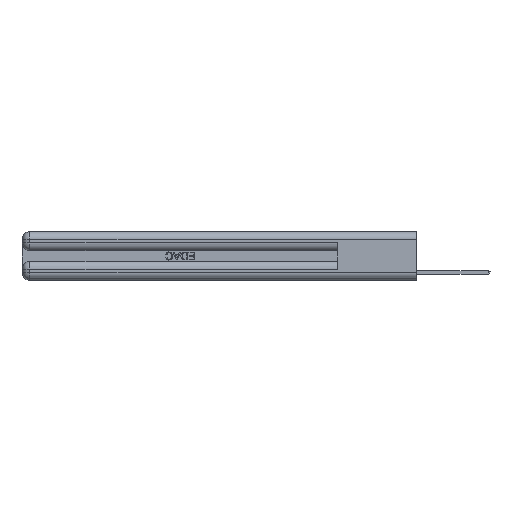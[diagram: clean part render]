
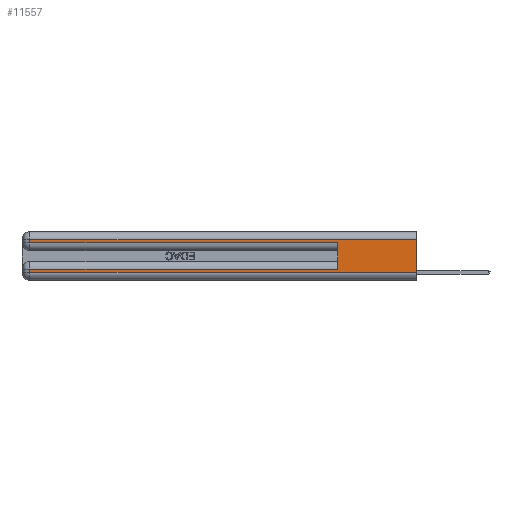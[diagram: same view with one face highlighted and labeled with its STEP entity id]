
A CAD part, left-side view. The second image highlights one B-rep face of the part: STEP entity #11557.
In plain terms, the highlighted planar face has unit normal (-1, 0, 0).
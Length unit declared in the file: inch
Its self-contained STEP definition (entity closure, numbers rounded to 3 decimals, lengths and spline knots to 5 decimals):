
#707 = EDGE_CURVE ( 'NONE', #21317, #33794, #14680, .T. ) ;
#1728 = LINE ( 'NONE', #34259, #22041 ) ;
#1925 = CARTESIAN_POINT ( 'NONE',  ( 0., 2.94, 0.31 ) ) ;
#2739 = VERTEX_POINT ( 'NONE', #4983 ) ;
#3100 = EDGE_CURVE ( 'NONE', #26718, #10492, #29266, .T. ) ;
#4014 = LINE ( 'NONE', #30188, #10774 ) ;
#4438 = CARTESIAN_POINT ( 'NONE',  ( 0., 0., 0.06 ) ) ;
#4591 = EDGE_CURVE ( 'NONE', #27402, #26718, #21952, .T. ) ;
#4983 = CARTESIAN_POINT ( 'NONE',  ( 0., 0., 0.31 ) ) ;
#5297 = VERTEX_POINT ( 'NONE', #15133 ) ;
#6548 = VECTOR ( 'NONE', #13263, 39.37008 ) ;
#7252 = DIRECTION ( 'NONE',  ( 0., 1., 0. ) ) ;
#7705 = CARTESIAN_POINT ( 'NONE',  ( 0., 0., 0.085 ) ) ;
#7969 = VECTOR ( 'NONE', #30083, 39.37008 ) ;
#8330 = VERTEX_POINT ( 'NONE', #4438 ) ;
#8535 = ORIENTED_EDGE ( 'NONE', *, *, #707, .T. ) ;
#8722 = EDGE_CURVE ( 'NONE', #2739, #8330, #13711, .T. ) ;
#8833 = DIRECTION ( 'NONE',  ( 0., 0., -1. ) ) ;
#8920 = ORIENTED_EDGE ( 'NONE', *, *, #8722, .F. ) ;
#9500 = CARTESIAN_POINT ( 'NONE',  ( 0., 2.94, 0.285 ) ) ;
#10492 = VERTEX_POINT ( 'NONE', #15556 ) ;
#10774 = VECTOR ( 'NONE', #32914, 39.37008 ) ;
#11097 = EDGE_CURVE ( 'NONE', #33794, #5297, #1728, .T. ) ;
#11557 = ADVANCED_FACE ( 'NONE', ( #16037 ), #32921, .F. ) ;
#12275 = EDGE_CURVE ( 'NONE', #27402, #5297, #18553, .T. ) ;
#13082 = CARTESIAN_POINT ( 'NONE',  ( 0., 2.94, 0.085 ) ) ;
#13263 = DIRECTION ( 'NONE',  ( 0., 0., -1. ) ) ;
#13315 = CARTESIAN_POINT ( 'NONE',  ( 0., 2.94, 0.37 ) ) ;
#13711 = LINE ( 'NONE', #34410, #6548 ) ;
#13886 = VECTOR ( 'NONE', #21706, 39.37008 ) ;
#14680 = LINE ( 'NONE', #24566, #7969 ) ;
#14850 = ORIENTED_EDGE ( 'NONE', *, *, #12275, .F. ) ;
#15133 = CARTESIAN_POINT ( 'NONE',  ( 0., 0.6, 0.285 ) ) ;
#15556 = CARTESIAN_POINT ( 'NONE',  ( 0., 2.94, 0.06 ) ) ;
#15573 = LINE ( 'NONE', #21485, #13886 ) ;
#15664 = DIRECTION ( 'NONE',  ( 0., 0., -1. ) ) ;
#16037 = FACE_OUTER_BOUND ( 'NONE', #33291, .T. ) ;
#16610 = CARTESIAN_POINT ( 'NONE',  ( 0., 0., 0.37 ) ) ;
#18553 = LINE ( 'NONE', #22605, #32613 ) ;
#19505 = VECTOR ( 'NONE', #15664, 39.37008 ) ;
#21317 = VERTEX_POINT ( 'NONE', #1925 ) ;
#21485 = CARTESIAN_POINT ( 'NONE',  ( 0., 0., 0.06 ) ) ;
#21706 = DIRECTION ( 'NONE',  ( 0., -1., 0. ) ) ;
#21952 = LINE ( 'NONE', #7705, #29655 ) ;
#22041 = VECTOR ( 'NONE', #25664, 39.37008 ) ;
#22192 = AXIS2_PLACEMENT_3D ( 'NONE', #16610, #22299, #8833 ) ;
#22299 = DIRECTION ( 'NONE',  ( 1., 0., 0. ) ) ;
#22605 = CARTESIAN_POINT ( 'NONE',  ( 0., 0.6, 0.145 ) ) ;
#23084 = ORIENTED_EDGE ( 'NONE', *, *, #25775, .T. ) ;
#24566 = CARTESIAN_POINT ( 'NONE',  ( 0., 2.94, 0.37 ) ) ;
#25339 = DIRECTION ( 'NONE',  ( 0., 0., 1. ) ) ;
#25664 = DIRECTION ( 'NONE',  ( 0., -1., 0. ) ) ;
#25775 = EDGE_CURVE ( 'NONE', #2739, #21317, #4014, .T. ) ;
#26470 = ORIENTED_EDGE ( 'NONE', *, *, #11097, .T. ) ;
#26718 = VERTEX_POINT ( 'NONE', #13082 ) ;
#27402 = VERTEX_POINT ( 'NONE', #28684 ) ;
#28146 = ORIENTED_EDGE ( 'NONE', *, *, #3100, .T. ) ;
#28684 = CARTESIAN_POINT ( 'NONE',  ( 0., 0.6, 0.085 ) ) ;
#29266 = LINE ( 'NONE', #13315, #19505 ) ;
#29655 = VECTOR ( 'NONE', #7252, 39.37008 ) ;
#30083 = DIRECTION ( 'NONE',  ( 0., 0., -1. ) ) ;
#30188 = CARTESIAN_POINT ( 'NONE',  ( 0., 0., 0.31 ) ) ;
#30344 = ORIENTED_EDGE ( 'NONE', *, *, #4591, .T. ) ;
#32079 = ORIENTED_EDGE ( 'NONE', *, *, #34830, .T. ) ;
#32613 = VECTOR ( 'NONE', #25339, 39.37008 ) ;
#32914 = DIRECTION ( 'NONE',  ( 0., 1., 0. ) ) ;
#32921 = PLANE ( 'NONE',  #22192 ) ;
#33291 = EDGE_LOOP ( 'NONE', ( #8920, #23084, #8535, #26470, #14850, #30344, #28146, #32079 ) ) ;
#33794 = VERTEX_POINT ( 'NONE', #9500 ) ;
#34259 = CARTESIAN_POINT ( 'NONE',  ( 0., 0., 0.285 ) ) ;
#34410 = CARTESIAN_POINT ( 'NONE',  ( 0., 0., 0.37 ) ) ;
#34830 = EDGE_CURVE ( 'NONE', #10492, #8330, #15573, .T. ) ;
